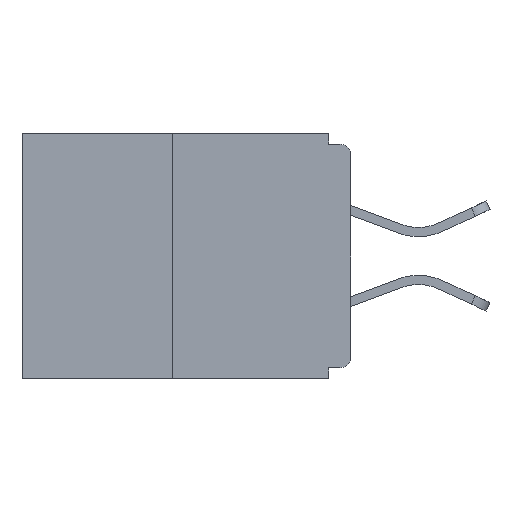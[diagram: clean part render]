
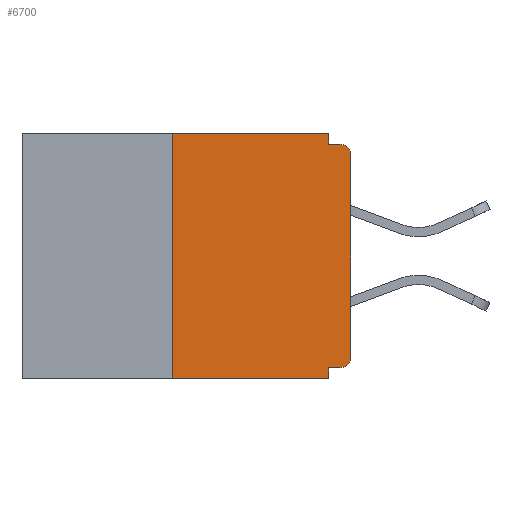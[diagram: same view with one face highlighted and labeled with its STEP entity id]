
A CAD part, left-side view. The second image highlights one B-rep face of the part: STEP entity #6700.
In plain terms, the highlighted planar face has unit normal (-1, 0, 0).
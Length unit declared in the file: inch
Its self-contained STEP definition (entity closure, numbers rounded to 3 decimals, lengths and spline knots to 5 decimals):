
#52 = VECTOR ( 'NONE', #10036, 39.37008 ) ;
#159 = EDGE_CURVE ( 'NONE', #12221, #4193, #4273, .T. ) ;
#457 = EDGE_CURVE ( 'NONE', #4193, #2254, #8086, .T. ) ;
#1084 = VERTEX_POINT ( 'NONE', #10756 ) ;
#1089 = ORIENTED_EDGE ( 'NONE', *, *, #2520, .F. ) ;
#1184 = VERTEX_POINT ( 'NONE', #1269 ) ;
#1269 = CARTESIAN_POINT ( 'NONE',  ( 0., 0.015, -0.015 ) ) ;
#1452 = LINE ( 'NONE', #14214, #7240 ) ;
#1637 = CIRCLE ( 'NONE', #14841, 0.015 ) ;
#1930 = ORIENTED_EDGE ( 'NONE', *, *, #4465, .T. ) ;
#2130 = VERTEX_POINT ( 'NONE', #3090 ) ;
#2254 = VERTEX_POINT ( 'NONE', #8642 ) ;
#2344 = VERTEX_POINT ( 'NONE', #4260 ) ;
#2351 = ORIENTED_EDGE ( 'NONE', *, *, #457, .F. ) ;
#2520 = EDGE_CURVE ( 'NONE', #14271, #7665, #7273, .T. ) ;
#2681 = DIRECTION ( 'NONE',  ( 0., -1., 0. ) ) ;
#2691 = VERTEX_POINT ( 'NONE', #4050 ) ;
#2866 = CARTESIAN_POINT ( 'NONE',  ( 0., 0.46, 0. ) ) ;
#3043 = DIRECTION ( 'NONE',  ( 0., 0., -1. ) ) ;
#3090 = CARTESIAN_POINT ( 'NONE',  ( 0., 0.25, -0.343 ) ) ;
#3739 = CARTESIAN_POINT ( 'NONE',  ( 0., 0.031, 0. ) ) ;
#3938 = ORIENTED_EDGE ( 'NONE', *, *, #5796, .T. ) ;
#4050 = CARTESIAN_POINT ( 'NONE',  ( 0., 0., -0.313 ) ) ;
#4124 = CARTESIAN_POINT ( 'NONE',  ( 0., 0.25, 0. ) ) ;
#4193 = VERTEX_POINT ( 'NONE', #14706 ) ;
#4260 = CARTESIAN_POINT ( 'NONE',  ( 0., 0., -0.03 ) ) ;
#4273 = LINE ( 'NONE', #8359, #10480 ) ;
#4366 = DIRECTION ( 'NONE',  ( -1., 0., 0. ) ) ;
#4465 = EDGE_CURVE ( 'NONE', #12221, #2691, #12992, .T. ) ;
#4755 = CARTESIAN_POINT ( 'NONE',  ( 0., 0.015, -0.313 ) ) ;
#4861 = DIRECTION ( 'NONE',  ( 0., 1., 0. ) ) ;
#4955 = VECTOR ( 'NONE', #3043, 39.37008 ) ;
#5106 = ORIENTED_EDGE ( 'NONE', *, *, #13711, .F. ) ;
#5489 = DIRECTION ( 'NONE',  ( 0., -1., 0. ) ) ;
#5796 = EDGE_CURVE ( 'NONE', #2691, #2344, #12784, .T. ) ;
#5828 = DIRECTION ( 'NONE',  ( 0., 0., -1. ) ) ;
#6700 = ADVANCED_FACE ( 'NONE', ( #13447 ), #9841, .F. ) ;
#7024 = ORIENTED_EDGE ( 'NONE', *, *, #7065, .T. ) ;
#7065 = EDGE_CURVE ( 'NONE', #2130, #2254, #13077, .T. ) ;
#7148 = ORIENTED_EDGE ( 'NONE', *, *, #159, .F. ) ;
#7184 = ORIENTED_EDGE ( 'NONE', *, *, #13428, .F. ) ;
#7240 = VECTOR ( 'NONE', #13001, 39.37008 ) ;
#7273 = LINE ( 'NONE', #11901, #12721 ) ;
#7665 = VERTEX_POINT ( 'NONE', #3739 ) ;
#8053 = CARTESIAN_POINT ( 'NONE',  ( 0., 0.031, 0. ) ) ;
#8086 = LINE ( 'NONE', #14748, #4955 ) ;
#8241 = VECTOR ( 'NONE', #10403, 39.37008 ) ;
#8359 = CARTESIAN_POINT ( 'NONE',  ( 0., 0., -0.328 ) ) ;
#8642 = CARTESIAN_POINT ( 'NONE',  ( 0., 0.031, -0.343 ) ) ;
#8672 = AXIS2_PLACEMENT_3D ( 'NONE', #2866, #10787, #11946 ) ;
#8811 = VECTOR ( 'NONE', #11756, 39.37008 ) ;
#8865 = ORIENTED_EDGE ( 'NONE', *, *, #12882, .T. ) ;
#9426 = DIRECTION ( 'NONE',  ( 0., 0., -1. ) ) ;
#9503 = CARTESIAN_POINT ( 'NONE',  ( 0., 0., 0. ) ) ;
#9841 = PLANE ( 'NONE',  #8672 ) ;
#10036 = DIRECTION ( 'NONE',  ( 0., 0., 1. ) ) ;
#10175 = CARTESIAN_POINT ( 'NONE',  ( 0., 0.015, -0.03 ) ) ;
#10403 = DIRECTION ( 'NONE',  ( 0., 0., -1. ) ) ;
#10480 = VECTOR ( 'NONE', #4861, 39.37008 ) ;
#10756 = CARTESIAN_POINT ( 'NONE',  ( 0., 0.031, -0.015 ) ) ;
#10787 = DIRECTION ( 'NONE',  ( 1., 0., 0. ) ) ;
#11283 = VECTOR ( 'NONE', #5489, 39.37008 ) ;
#11362 = EDGE_CURVE ( 'NONE', #7665, #1084, #12183, .T. ) ;
#11597 = ORIENTED_EDGE ( 'NONE', *, *, #11362, .F. ) ;
#11681 = DIRECTION ( 'NONE',  ( -1., 0., 0. ) ) ;
#11756 = DIRECTION ( 'NONE',  ( 0., 0., 1. ) ) ;
#11901 = CARTESIAN_POINT ( 'NONE',  ( 0., 0.46, 0. ) ) ;
#11946 = DIRECTION ( 'NONE',  ( 0., 0., -1. ) ) ;
#11970 = LINE ( 'NONE', #4124, #52 ) ;
#12183 = LINE ( 'NONE', #8053, #8241 ) ;
#12221 = VERTEX_POINT ( 'NONE', #14634 ) ;
#12721 = VECTOR ( 'NONE', #2681, 39.37008 ) ;
#12784 = LINE ( 'NONE', #9503, #8811 ) ;
#12882 = EDGE_CURVE ( 'NONE', #2344, #1184, #1637, .T. ) ;
#12992 = CIRCLE ( 'NONE', #14896, 0.015 ) ;
#13001 = DIRECTION ( 'NONE',  ( 0., -1., 0. ) ) ;
#13077 = LINE ( 'NONE', #14744, #11283 ) ;
#13428 = EDGE_CURVE ( 'NONE', #1084, #1184, #1452, .T. ) ;
#13447 = FACE_OUTER_BOUND ( 'NONE', #14403, .T. ) ;
#13711 = EDGE_CURVE ( 'NONE', #2130, #14271, #11970, .T. ) ;
#14214 = CARTESIAN_POINT ( 'NONE',  ( 0., 0., -0.015 ) ) ;
#14271 = VERTEX_POINT ( 'NONE', #14284 ) ;
#14284 = CARTESIAN_POINT ( 'NONE',  ( 0., 0.25, 0. ) ) ;
#14403 = EDGE_LOOP ( 'NONE', ( #1089, #5106, #7024, #2351, #7148, #1930, #3938, #8865, #7184, #11597 ) ) ;
#14634 = CARTESIAN_POINT ( 'NONE',  ( 0., 0.015, -0.328 ) ) ;
#14706 = CARTESIAN_POINT ( 'NONE',  ( 0., 0.031, -0.328 ) ) ;
#14744 = CARTESIAN_POINT ( 'NONE',  ( 0., 0.46, -0.343 ) ) ;
#14748 = CARTESIAN_POINT ( 'NONE',  ( 0., 0.031, -0.343 ) ) ;
#14841 = AXIS2_PLACEMENT_3D ( 'NONE', #10175, #4366, #9426 ) ;
#14896 = AXIS2_PLACEMENT_3D ( 'NONE', #4755, #11681, #5828 ) ;
